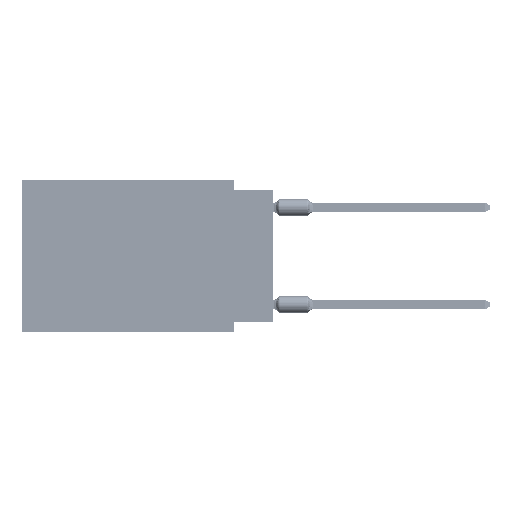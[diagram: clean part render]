
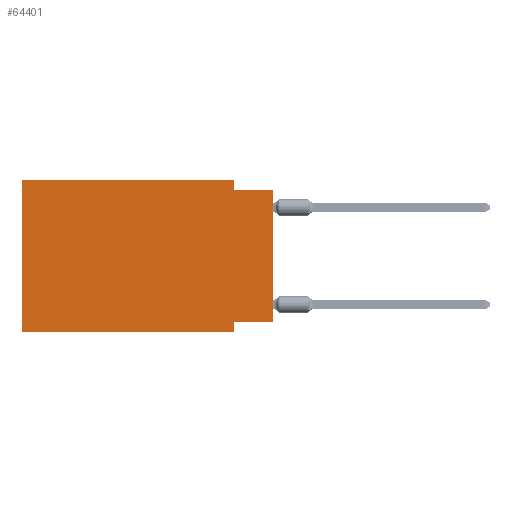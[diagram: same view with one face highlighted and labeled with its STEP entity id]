
A CAD part, left-side view. The second image highlights one B-rep face of the part: STEP entity #64401.
In plain terms, the highlighted planar face has unit normal (-1, 0, 0).
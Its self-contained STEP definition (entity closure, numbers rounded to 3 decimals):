
#1263 = ORIENTED_EDGE ( 'NONE', *, *, #23555, .F. ) ;
#1470 = VERTEX_POINT ( 'NONE', #70052 ) ;
#2712 = ORIENTED_EDGE ( 'NONE', *, *, #69484, .F. ) ;
#5224 = VECTOR ( 'NONE', #52043, 1000. ) ;
#5708 = VECTOR ( 'NONE', #19962, 1000. ) ;
#6013 = CARTESIAN_POINT ( 'NONE',  ( 0., 2.54, -9.906 ) ) ;
#7869 = LINE ( 'NONE', #42258, #16047 ) ;
#8153 = ORIENTED_EDGE ( 'NONE', *, *, #45556, .T. ) ;
#10228 = DIRECTION ( 'NONE',  ( 0., -1., 0. ) ) ;
#11464 = EDGE_LOOP ( 'NONE', ( #8153, #2712, #39183, #55276, #1263, #73054, #40971, #15447 ) ) ;
#13410 = CARTESIAN_POINT ( 'NONE',  ( 0., 0., 0. ) ) ;
#14268 = CARTESIAN_POINT ( 'NONE',  ( 0., 2.54, 0. ) ) ;
#15447 = ORIENTED_EDGE ( 'NONE', *, *, #71704, .F. ) ;
#16047 = VECTOR ( 'NONE', #29822, 1000. ) ;
#16941 = CARTESIAN_POINT ( 'NONE',  ( 0., 0., -0.635 ) ) ;
#17893 = CARTESIAN_POINT ( 'NONE',  ( 0., 16.383, 0. ) ) ;
#18776 = VECTOR ( 'NONE', #63176, 1000. ) ;
#19962 = DIRECTION ( 'NONE',  ( 0., 0., -1. ) ) ;
#22068 = VECTOR ( 'NONE', #10228, 1000. ) ;
#23555 = EDGE_CURVE ( 'NONE', #27878, #39803, #59015, .T. ) ;
#27878 = VERTEX_POINT ( 'NONE', #61143 ) ;
#29822 = DIRECTION ( 'NONE',  ( 0., -1., 0. ) ) ;
#32386 = CARTESIAN_POINT ( 'NONE',  ( 0., 0., -0.635 ) ) ;
#35023 = PLANE ( 'NONE',  #64404 ) ;
#35128 = VECTOR ( 'NONE', #37293, 1000. ) ;
#35336 = EDGE_CURVE ( 'NONE', #39803, #48485, #7869, .T. ) ;
#35527 = CARTESIAN_POINT ( 'NONE',  ( 0., 2.54, -9.271 ) ) ;
#35753 = CARTESIAN_POINT ( 'NONE',  ( 0., 16.383, 0. ) ) ;
#36099 = VECTOR ( 'NONE', #71067, 1000. ) ;
#36134 = DIRECTION ( 'NONE',  ( 1., 0., 0. ) ) ;
#36586 = LINE ( 'NONE', #54688, #5708 ) ;
#36914 = LINE ( 'NONE', #14268, #35128 ) ;
#37293 = DIRECTION ( 'NONE',  ( 0., 0., -1. ) ) ;
#39183 = ORIENTED_EDGE ( 'NONE', *, *, #45212, .F. ) ;
#39541 = CARTESIAN_POINT ( 'NONE',  ( 0., 16.383, 0. ) ) ;
#39803 = VERTEX_POINT ( 'NONE', #39541 ) ;
#40176 = CARTESIAN_POINT ( 'NONE',  ( 0., 0., -9.271 ) ) ;
#40971 = ORIENTED_EDGE ( 'NONE', *, *, #40973, .F. ) ;
#40973 = EDGE_CURVE ( 'NONE', #72235, #52461, #36586, .T. ) ;
#42258 = CARTESIAN_POINT ( 'NONE',  ( 0., 16.383, 0. ) ) ;
#42395 = VECTOR ( 'NONE', #66242, 1000. ) ;
#45212 = EDGE_CURVE ( 'NONE', #48485, #1470, #36914, .T. ) ;
#45556 = EDGE_CURVE ( 'NONE', #52633, #48941, #64741, .T. ) ;
#48485 = VERTEX_POINT ( 'NONE', #60383 ) ;
#48941 = VERTEX_POINT ( 'NONE', #32386 ) ;
#51670 = LINE ( 'NONE', #16941, #5224 ) ;
#52043 = DIRECTION ( 'NONE',  ( 0., -1., 0. ) ) ;
#52461 = VERTEX_POINT ( 'NONE', #6013 ) ;
#52633 = VERTEX_POINT ( 'NONE', #59218 ) ;
#54688 = CARTESIAN_POINT ( 'NONE',  ( 0., 2.54, -9.906 ) ) ;
#55276 = ORIENTED_EDGE ( 'NONE', *, *, #35336, .F. ) ;
#58401 = DIRECTION ( 'NONE',  ( 0., 0., -1. ) ) ;
#59015 = LINE ( 'NONE', #17893, #36099 ) ;
#59218 = CARTESIAN_POINT ( 'NONE',  ( 0., 0., -9.271 ) ) ;
#60383 = CARTESIAN_POINT ( 'NONE',  ( 0., 2.54, 0. ) ) ;
#61143 = CARTESIAN_POINT ( 'NONE',  ( 0., 16.383, -9.906 ) ) ;
#61208 = CARTESIAN_POINT ( 'NONE',  ( 0., 16.383, -9.906 ) ) ;
#63176 = DIRECTION ( 'NONE',  ( 0., 1., 0. ) ) ;
#63551 = LINE ( 'NONE', #40176, #18776 ) ;
#64401 = ADVANCED_FACE ( 'NONE', ( #64790 ), #35023, .F. ) ;
#64404 = AXIS2_PLACEMENT_3D ( 'NONE', #35753, #36134, #58401 ) ;
#64741 = LINE ( 'NONE', #13410, #42395 ) ;
#64790 = FACE_OUTER_BOUND ( 'NONE', #11464, .T. ) ;
#66242 = DIRECTION ( 'NONE',  ( 0., 0., 1. ) ) ;
#69014 = EDGE_CURVE ( 'NONE', #27878, #52461, #72902, .T. ) ;
#69484 = EDGE_CURVE ( 'NONE', #1470, #48941, #51670, .T. ) ;
#70052 = CARTESIAN_POINT ( 'NONE',  ( 0., 2.54, -0.635 ) ) ;
#71067 = DIRECTION ( 'NONE',  ( 0., 0., 1. ) ) ;
#71704 = EDGE_CURVE ( 'NONE', #52633, #72235, #63551, .T. ) ;
#72235 = VERTEX_POINT ( 'NONE', #35527 ) ;
#72902 = LINE ( 'NONE', #61208, #22068 ) ;
#73054 = ORIENTED_EDGE ( 'NONE', *, *, #69014, .T. ) ;
